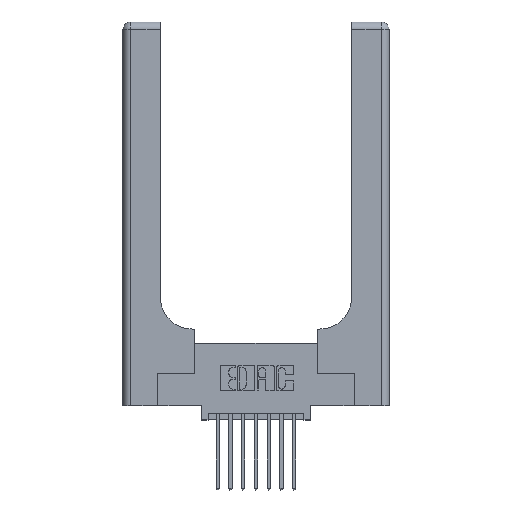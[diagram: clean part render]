
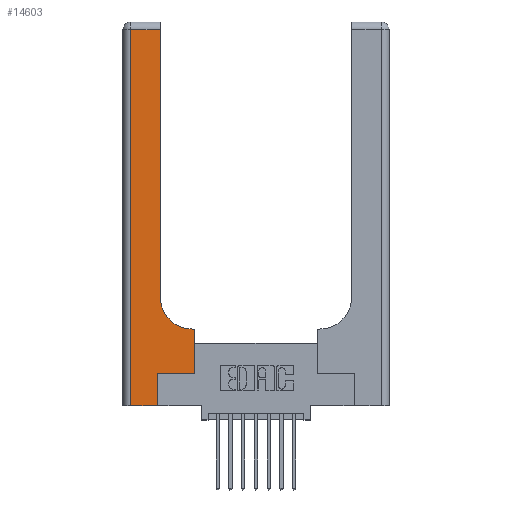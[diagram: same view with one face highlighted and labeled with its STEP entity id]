
A CAD part, top view. The second image highlights one B-rep face of the part: STEP entity #14603.
In plain terms, the highlighted planar face has unit normal (0, 0, 1).
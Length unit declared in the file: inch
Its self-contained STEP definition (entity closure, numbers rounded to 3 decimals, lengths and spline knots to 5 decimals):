
#48 = PLANE ( 'NONE',  #8110 ) ;
#147 = CARTESIAN_POINT ( 'NONE',  ( 0., 2.94, 0.37 ) ) ;
#348 = EDGE_CURVE ( 'NONE', #8730, #12559, #15402, .T. ) ;
#483 = EDGE_CURVE ( 'NONE', #2264, #8876, #5420, .T. ) ;
#587 = ORIENTED_EDGE ( 'NONE', *, *, #6184, .T. ) ;
#1288 = CARTESIAN_POINT ( 'NONE',  ( 0.269, 0.25, 0.37 ) ) ;
#1312 = DIRECTION ( 'NONE',  ( 0., 0., -1. ) ) ;
#1509 = CARTESIAN_POINT ( 'NONE',  ( 0.2915, 2.94, 0.37 ) ) ;
#1589 = DIRECTION ( 'NONE',  ( 0., 1., 0. ) ) ;
#1789 = CARTESIAN_POINT ( 'NONE',  ( 0.5585, 0.25, 0.37 ) ) ;
#1812 = AXIS2_PLACEMENT_3D ( 'NONE', #14926, #5243, #7638 ) ;
#1966 = CARTESIAN_POINT ( 'NONE',  ( 0.269, 0.25, 0.37 ) ) ;
#1994 = ORIENTED_EDGE ( 'NONE', *, *, #12052, .T. ) ;
#2015 = EDGE_CURVE ( 'NONE', #10128, #2123, #8605, .T. ) ;
#2123 = VERTEX_POINT ( 'NONE', #8912 ) ;
#2264 = VERTEX_POINT ( 'NONE', #9398 ) ;
#2741 = ORIENTED_EDGE ( 'NONE', *, *, #14974, .T. ) ;
#3571 = CARTESIAN_POINT ( 'NONE',  ( 0., 3., 0.37 ) ) ;
#3879 = CARTESIAN_POINT ( 'NONE',  ( 0.2915, 0.6, 0.37 ) ) ;
#3891 = CARTESIAN_POINT ( 'NONE',  ( 0.269, 0., 0.37 ) ) ;
#3942 = CARTESIAN_POINT ( 'NONE',  ( 0.5415, 0.6, 0.37 ) ) ;
#4260 = ORIENTED_EDGE ( 'NONE', *, *, #2015, .T. ) ;
#4824 = ORIENTED_EDGE ( 'NONE', *, *, #348, .T. ) ;
#5156 = EDGE_CURVE ( 'NONE', #8876, #5649, #13771, .T. ) ;
#5243 = DIRECTION ( 'NONE',  ( 0., 0., -1. ) ) ;
#5382 = LINE ( 'NONE', #3891, #6714 ) ;
#5420 = LINE ( 'NONE', #3879, #7503 ) ;
#5422 = DIRECTION ( 'NONE',  ( 0., 1., 0. ) ) ;
#5649 = VERTEX_POINT ( 'NONE', #7211 ) ;
#6184 = EDGE_CURVE ( 'NONE', #5649, #10128, #6510, .T. ) ;
#6510 = LINE ( 'NONE', #8553, #9881 ) ;
#6714 = VECTOR ( 'NONE', #8474, 39.37008 ) ;
#7211 = CARTESIAN_POINT ( 'NONE',  ( 0.2915, 0.85, 0.37 ) ) ;
#7503 = VECTOR ( 'NONE', #13187, 39.37008 ) ;
#7542 = ORIENTED_EDGE ( 'NONE', *, *, #13442, .T. ) ;
#7638 = DIRECTION ( 'NONE',  ( 1., 0., 0. ) ) ;
#7845 = CARTESIAN_POINT ( 'NONE',  ( 0.269, 0., 0.37 ) ) ;
#8004 = CARTESIAN_POINT ( 'NONE',  ( 0.06, 0., 0.37 ) ) ;
#8110 = AXIS2_PLACEMENT_3D ( 'NONE', #3571, #1312, #9561 ) ;
#8166 = EDGE_LOOP ( 'NONE', ( #587, #4260, #7542, #8685, #1994, #4824, #2741, #11350, #8608 ) ) ;
#8398 = VERTEX_POINT ( 'NONE', #7845 ) ;
#8474 = DIRECTION ( 'NONE',  ( 0., 1., 0. ) ) ;
#8479 = CARTESIAN_POINT ( 'NONE',  ( 0., 0., 0.37 ) ) ;
#8553 = CARTESIAN_POINT ( 'NONE',  ( 0.2915, 3., 0.37 ) ) ;
#8565 = VERTEX_POINT ( 'NONE', #8004 ) ;
#8605 = LINE ( 'NONE', #147, #9380 ) ;
#8608 = ORIENTED_EDGE ( 'NONE', *, *, #5156, .T. ) ;
#8685 = ORIENTED_EDGE ( 'NONE', *, *, #13535, .T. ) ;
#8730 = VERTEX_POINT ( 'NONE', #1288 ) ;
#8876 = VERTEX_POINT ( 'NONE', #3942 ) ;
#8912 = CARTESIAN_POINT ( 'NONE',  ( 0.06, 2.94, 0.37 ) ) ;
#8927 = VECTOR ( 'NONE', #14256, 39.37008 ) ;
#9380 = VECTOR ( 'NONE', #11014, 39.37008 ) ;
#9398 = CARTESIAN_POINT ( 'NONE',  ( 0.5585, 0.6, 0.37 ) ) ;
#9561 = DIRECTION ( 'NONE',  ( -1., 0., 0. ) ) ;
#9881 = VECTOR ( 'NONE', #1589, 39.37008 ) ;
#10128 = VERTEX_POINT ( 'NONE', #1509 ) ;
#10629 = LINE ( 'NONE', #8479, #12892 ) ;
#10800 = CARTESIAN_POINT ( 'NONE',  ( 0.06, 3., 0.37 ) ) ;
#10846 = DIRECTION ( 'NONE',  ( 1., 0., 0. ) ) ;
#11014 = DIRECTION ( 'NONE',  ( -1., 0., 0. ) ) ;
#11350 = ORIENTED_EDGE ( 'NONE', *, *, #483, .T. ) ;
#11380 = LINE ( 'NONE', #10800, #8927 ) ;
#12052 = EDGE_CURVE ( 'NONE', #8398, #8730, #5382, .T. ) ;
#12459 = VECTOR ( 'NONE', #5422, 39.37008 ) ;
#12559 = VERTEX_POINT ( 'NONE', #15394 ) ;
#12681 = DIRECTION ( 'NONE',  ( 1., 0., 0. ) ) ;
#12892 = VECTOR ( 'NONE', #10846, 39.37008 ) ;
#13187 = DIRECTION ( 'NONE',  ( -1., 0., 0. ) ) ;
#13442 = EDGE_CURVE ( 'NONE', #2123, #8565, #11380, .T. ) ;
#13535 = EDGE_CURVE ( 'NONE', #8565, #8398, #10629, .T. ) ;
#13771 = CIRCLE ( 'NONE', #1812, 0.25 ) ;
#14256 = DIRECTION ( 'NONE',  ( 0., -1., 0. ) ) ;
#14266 = VECTOR ( 'NONE', #12681, 39.37008 ) ;
#14603 = ADVANCED_FACE ( 'NONE', ( #15466 ), #48, .F. ) ;
#14926 = CARTESIAN_POINT ( 'NONE',  ( 0.5415, 0.85, 0.37 ) ) ;
#14974 = EDGE_CURVE ( 'NONE', #12559, #2264, #15071, .T. ) ;
#15071 = LINE ( 'NONE', #1789, #12459 ) ;
#15394 = CARTESIAN_POINT ( 'NONE',  ( 0.5585, 0.25, 0.37 ) ) ;
#15402 = LINE ( 'NONE', #1966, #14266 ) ;
#15466 = FACE_OUTER_BOUND ( 'NONE', #8166, .T. ) ;
